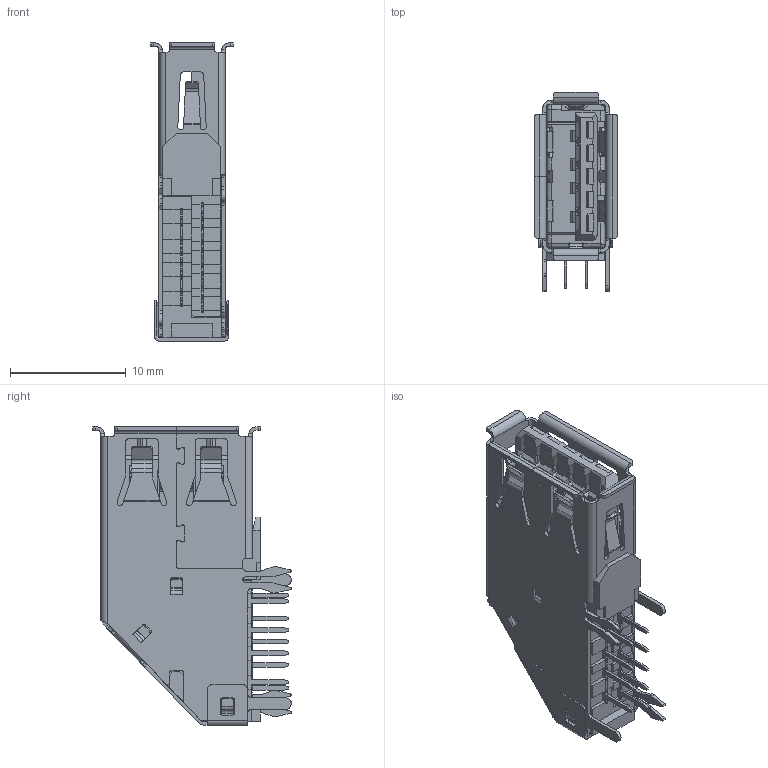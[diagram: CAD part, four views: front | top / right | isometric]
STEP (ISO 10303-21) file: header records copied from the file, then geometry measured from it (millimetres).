
FILE_DESCRIPTION (( 'STEP AP214' ), '1' );
FILE_NAME ('690D109-139-012.STEP', '2021-01-14T17:49:46', ( '' ), ( '' ), 'SwSTEP 2.0', 'SolidWorks 2020', '' );
FILE_SCHEMA (( 'AUTOMOTIVE_DESIGN' ));
Length unit declared in the file: millimetre
Products named in the file (14): Contact 2.0 1 690D109-X39-0XX; Contact 2.0 2 690D109-X39-0XX; Insulator 1 690D109-X39-0XX_Blue; 690D109-139-012; Shell 2 690D109-X39-0XX; Contact 3.0 9 690D109-X39-0XX; Contact 3.0 6 690D109-X39-0XX; Contact 3.0 5 690D109-X39-0XX; Contact 3.0 7 690D109-X39-0XX; Insulator 2 690D109-X39-0XX_Blue; Contact 2.0 4 690D109-X39-0XX; Shell 1 690D109-X39-0XX; Contact 3.0 8 690D109-X39-0XX; Contact 2.0 3 690D109-X39-0XX
Assembly tree (13 placements, depth 2):
  690D109-139-012
    Insulator 1 690D109-X39-0XX_Blue
    Contact 3.0 5 690D109-X39-0XX
    Contact 3.0 6 690D109-X39-0XX
    Contact 3.0 7 690D109-X39-0XX
    Contact 3.0 8 690D109-X39-0XX
    Contact 3.0 9 690D109-X39-0XX
    Insulator 2 690D109-X39-0XX_Blue
    Contact 2.0 1 690D109-X39-0XX
    Contact 2.0 2 690D109-X39-0XX
    Contact 2.0 3 690D109-X39-0XX
    Contact 2.0 4 690D109-X39-0XX
    Shell 1 690D109-X39-0XX
    Shell 2 690D109-X39-0XX
Bounding box: 7.12 x 17.16 x 25.75 mm (x, y, z)
Volume: 1029.9 mm3; surface area: 4329.4 mm2
Topology: 13 solids, 13 shells, 2780 faces, 8220 edges, 5346 vertices
Faces by surface type: plane 1938, cylinder 770, cone 37, bspline 35
Entity records: 94290 total; most frequent: CARTESIAN_POINT 19521, ORIENTED_EDGE 16436, DIRECTION 14415, EDGE_CURVE 8218, VECTOR 6213, LINE 6213, VERTEX_POINT 5346, AXIS2_PLACEMENT_3D 4101
